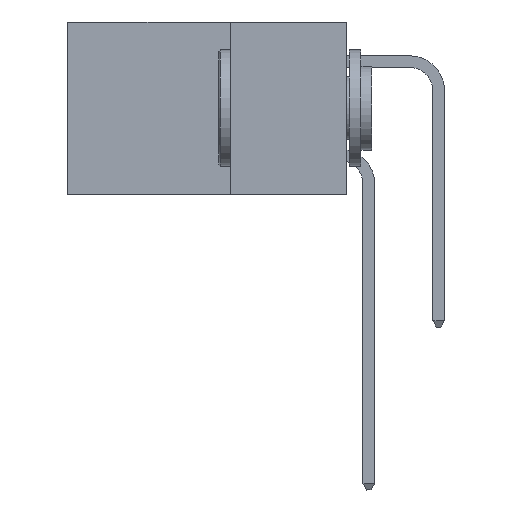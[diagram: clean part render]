
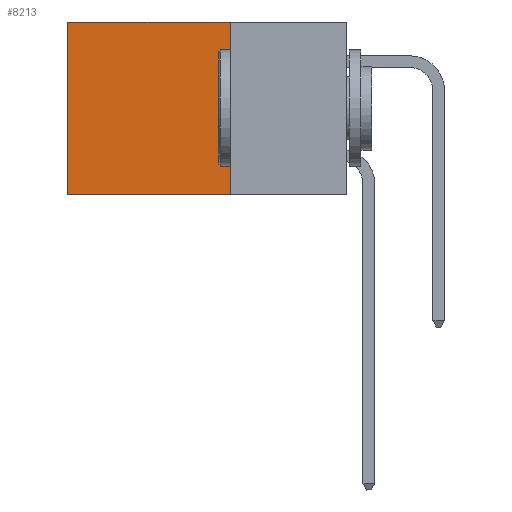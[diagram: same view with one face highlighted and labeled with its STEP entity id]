
A CAD part, left-side view. The second image highlights one B-rep face of the part: STEP entity #8213.
In plain terms, the highlighted planar face has unit normal (-1, 0, 0).
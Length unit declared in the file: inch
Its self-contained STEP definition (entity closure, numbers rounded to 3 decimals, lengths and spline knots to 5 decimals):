
#820 = ORIENTED_EDGE ( 'NONE', *, *, #4673, .T. ) ;
#846 = LINE ( 'NONE', #13637, #16438 ) ;
#1303 = LINE ( 'NONE', #11349, #8198 ) ;
#2344 = ORIENTED_EDGE ( 'NONE', *, *, #6332, .F. ) ;
#2688 = ORIENTED_EDGE ( 'NONE', *, *, #11552, .F. ) ;
#3223 = DIRECTION ( 'NONE',  ( 0., 1., 0. ) ) ;
#3602 = ORIENTED_EDGE ( 'NONE', *, *, #16073, .T. ) ;
#4673 = EDGE_CURVE ( 'NONE', #5434, #10664, #1303, .T. ) ;
#5434 = VERTEX_POINT ( 'NONE', #7646 ) ;
#5453 = CARTESIAN_POINT ( 'NONE',  ( 0.2875, 0.25, -0.37 ) ) ;
#5902 = DIRECTION ( 'NONE',  ( 1., 0., 0. ) ) ;
#6332 = EDGE_CURVE ( 'NONE', #12570, #10201, #11919, .T. ) ;
#6937 = LINE ( 'NONE', #15889, #9901 ) ;
#7646 = CARTESIAN_POINT ( 'NONE',  ( 0.2875, 0.25, 0. ) ) ;
#8135 = VECTOR ( 'NONE', #3223, 39.37008 ) ;
#8198 = VECTOR ( 'NONE', #12573, 39.37008 ) ;
#8213 = ADVANCED_FACE ( 'NONE', ( #11292 ), #15804, .F. ) ;
#9901 = VECTOR ( 'NONE', #11059, 39.37008 ) ;
#10201 = VERTEX_POINT ( 'NONE', #13185 ) ;
#10664 = VERTEX_POINT ( 'NONE', #11642 ) ;
#10956 = CARTESIAN_POINT ( 'NONE',  ( 0.2875, 0.25, 0. ) ) ;
#11059 = DIRECTION ( 'NONE',  ( 0., 0., -1. ) ) ;
#11292 = FACE_OUTER_BOUND ( 'NONE', #12489, .T. ) ;
#11349 = CARTESIAN_POINT ( 'NONE',  ( 0.2875, 0.25, 0. ) ) ;
#11552 = EDGE_CURVE ( 'NONE', #5434, #12570, #6937, .T. ) ;
#11642 = CARTESIAN_POINT ( 'NONE',  ( 0.2875, 0.6, 0. ) ) ;
#11919 = LINE ( 'NONE', #15749, #8135 ) ;
#12489 = EDGE_LOOP ( 'NONE', ( #3602, #2344, #2688, #820 ) ) ;
#12529 = AXIS2_PLACEMENT_3D ( 'NONE', #10956, #5902, #14647 ) ;
#12570 = VERTEX_POINT ( 'NONE', #5453 ) ;
#12573 = DIRECTION ( 'NONE',  ( 0., 1., 0. ) ) ;
#13185 = CARTESIAN_POINT ( 'NONE',  ( 0.2875, 0.6, -0.37 ) ) ;
#13637 = CARTESIAN_POINT ( 'NONE',  ( 0.2875, 0.6, 0. ) ) ;
#14647 = DIRECTION ( 'NONE',  ( 0., 0., -1. ) ) ;
#14839 = DIRECTION ( 'NONE',  ( 0., 0., -1. ) ) ;
#15749 = CARTESIAN_POINT ( 'NONE',  ( 0.2875, 0.25, -0.37 ) ) ;
#15804 = PLANE ( 'NONE',  #12529 ) ;
#15889 = CARTESIAN_POINT ( 'NONE',  ( 0.2875, 0.25, 0. ) ) ;
#16073 = EDGE_CURVE ( 'NONE', #10664, #10201, #846, .T. ) ;
#16438 = VECTOR ( 'NONE', #14839, 39.37008 ) ;
